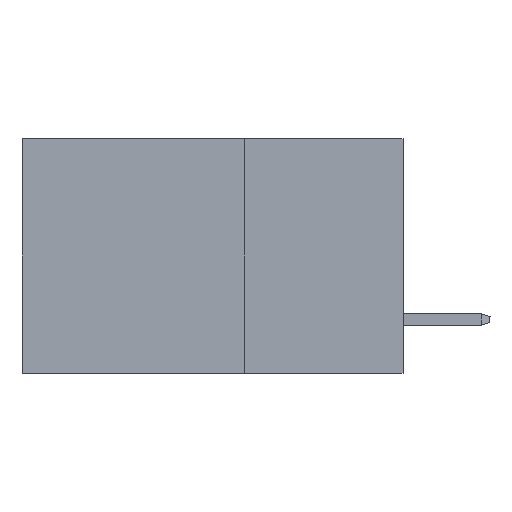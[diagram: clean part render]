
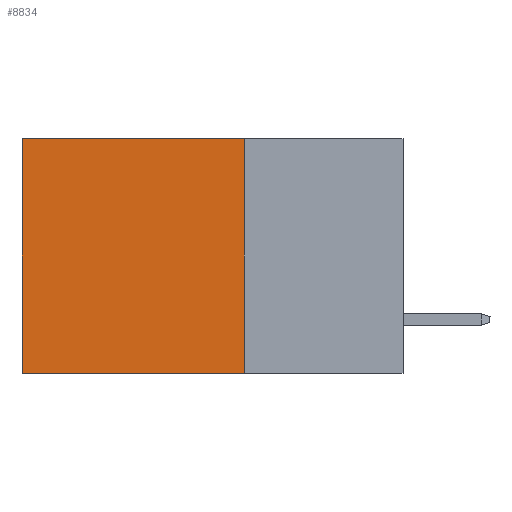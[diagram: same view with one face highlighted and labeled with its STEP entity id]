
A CAD part, left-side view. The second image highlights one B-rep face of the part: STEP entity #8834.
In plain terms, the highlighted planar face has unit normal (-1, 0, 0).
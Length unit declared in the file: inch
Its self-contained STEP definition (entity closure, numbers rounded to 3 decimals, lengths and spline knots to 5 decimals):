
#898 = DIRECTION ( 'NONE',  ( 1., 0., 0. ) ) ;
#1057 = EDGE_CURVE ( 'NONE', #6622, #5287, #17876, .T. ) ;
#2237 = DIRECTION ( 'NONE',  ( 0., 1., 0. ) ) ;
#2764 = EDGE_CURVE ( 'NONE', #11874, #6622, #15193, .T. ) ;
#4547 = CARTESIAN_POINT ( 'NONE',  ( 0.2875, 0.25, 0. ) ) ;
#4886 = CARTESIAN_POINT ( 'NONE',  ( 0.2875, 0.25, -0.37 ) ) ;
#5287 = VERTEX_POINT ( 'NONE', #13179 ) ;
#5986 = VECTOR ( 'NONE', #13569, 39.37008 ) ;
#6454 = CARTESIAN_POINT ( 'NONE',  ( 0.2875, 0.25, 0. ) ) ;
#6622 = VERTEX_POINT ( 'NONE', #4886 ) ;
#6939 = EDGE_CURVE ( 'NONE', #11874, #22822, #24826, .T. ) ;
#7087 = VECTOR ( 'NONE', #19994, 39.37008 ) ;
#7515 = CARTESIAN_POINT ( 'NONE',  ( 0.2875, 0.6, 0. ) ) ;
#8251 = ORIENTED_EDGE ( 'NONE', *, *, #16172, .T. ) ;
#8420 = ORIENTED_EDGE ( 'NONE', *, *, #1057, .F. ) ;
#8834 = ADVANCED_FACE ( 'NONE', ( #12707 ), #25871, .F. ) ;
#8861 = CARTESIAN_POINT ( 'NONE',  ( 0.2875, 0.25, 0. ) ) ;
#9011 = CARTESIAN_POINT ( 'NONE',  ( 0.2875, 0.25, -0.37 ) ) ;
#11874 = VERTEX_POINT ( 'NONE', #6454 ) ;
#12707 = FACE_OUTER_BOUND ( 'NONE', #23871, .T. ) ;
#13179 = CARTESIAN_POINT ( 'NONE',  ( 0.2875, 0.6, -0.37 ) ) ;
#13569 = DIRECTION ( 'NONE',  ( 0., 0., -1. ) ) ;
#14626 = DIRECTION ( 'NONE',  ( 0., 0., -1. ) ) ;
#15193 = LINE ( 'NONE', #4547, #5986 ) ;
#15547 = LINE ( 'NONE', #7515, #7087 ) ;
#16172 = EDGE_CURVE ( 'NONE', #22822, #5287, #15547, .T. ) ;
#17876 = LINE ( 'NONE', #9011, #29082 ) ;
#19666 = ORIENTED_EDGE ( 'NONE', *, *, #6939, .T. ) ;
#19994 = DIRECTION ( 'NONE',  ( 0., 0., -1. ) ) ;
#21077 = ORIENTED_EDGE ( 'NONE', *, *, #2764, .F. ) ;
#22730 = DIRECTION ( 'NONE',  ( 0., 1., 0. ) ) ;
#22822 = VERTEX_POINT ( 'NONE', #24101 ) ;
#23636 = VECTOR ( 'NONE', #22730, 39.37008 ) ;
#23871 = EDGE_LOOP ( 'NONE', ( #8251, #8420, #21077, #19666 ) ) ;
#24101 = CARTESIAN_POINT ( 'NONE',  ( 0.2875, 0.6, 0. ) ) ;
#24199 = AXIS2_PLACEMENT_3D ( 'NONE', #27951, #898, #14626 ) ;
#24826 = LINE ( 'NONE', #8861, #23636 ) ;
#25871 = PLANE ( 'NONE',  #24199 ) ;
#27951 = CARTESIAN_POINT ( 'NONE',  ( 0.2875, 0.25, 0. ) ) ;
#29082 = VECTOR ( 'NONE', #2237, 39.37008 ) ;
